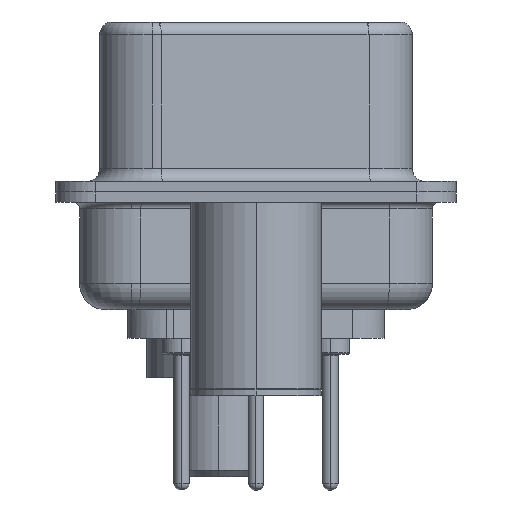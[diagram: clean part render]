
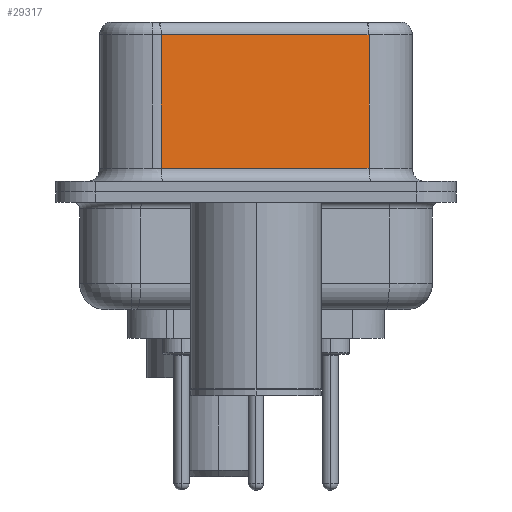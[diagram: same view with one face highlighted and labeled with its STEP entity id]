
A CAD part, left-side view. The second image highlights one B-rep face of the part: STEP entity #29317.
In plain terms, the highlighted planar face has unit normal (-0.985, -0.174, 0).
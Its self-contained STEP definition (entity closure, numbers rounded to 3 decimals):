
#489 = EDGE_CURVE ( 'NONE', #21842, #25849, #25945, .T. ) ;
#1246 = LINE ( 'NONE', #29912, #21366 ) ;
#1677 = ORIENTED_EDGE ( 'NONE', *, *, #489, .T. ) ;
#4131 = CARTESIAN_POINT ( 'NONE',  ( 5.132, -4.322, 6.52 ) ) ;
#5094 = VECTOR ( 'NONE', #27784, 1000. ) ;
#6689 = PLANE ( 'NONE',  #12031 ) ;
#7883 = DIRECTION ( 'NONE',  ( -0.174, 0.985, 0. ) ) ;
#8795 = ORIENTED_EDGE ( 'NONE', *, *, #30338, .T. ) ;
#10696 = EDGE_LOOP ( 'NONE', ( #17632, #11243, #1677, #8795 ) ) ;
#11243 = ORIENTED_EDGE ( 'NONE', *, *, #29859, .T. ) ;
#11762 = DIRECTION ( 'NONE',  ( -0.174, 0.985, 0. ) ) ;
#12031 = AXIS2_PLACEMENT_3D ( 'NONE', #4131, #26815, #11762 ) ;
#12328 = DIRECTION ( 'NONE',  ( 0.174, -0.985, 0. ) ) ;
#12344 = VECTOR ( 'NONE', #7883, 1000. ) ;
#14099 = DIRECTION ( 'NONE',  ( 0., 0., -1. ) ) ;
#14786 = VECTOR ( 'NONE', #14099, 1000. ) ;
#14796 = CARTESIAN_POINT ( 'NONE',  ( 3.73, 3.628, 0.9 ) ) ;
#17632 = ORIENTED_EDGE ( 'NONE', *, *, #28607, .F. ) ;
#17885 = CARTESIAN_POINT ( 'NONE',  ( 3.73, 3.628, 6.02 ) ) ;
#18937 = VERTEX_POINT ( 'NONE', #21429 ) ;
#19821 = LINE ( 'NONE', #27975, #12344 ) ;
#21366 = VECTOR ( 'NONE', #12328, 1000. ) ;
#21429 = CARTESIAN_POINT ( 'NONE',  ( 5.132, -4.322, 0.9 ) ) ;
#21842 = VERTEX_POINT ( 'NONE', #17885 ) ;
#22849 = CARTESIAN_POINT ( 'NONE',  ( 3.73, 3.628, 6.52 ) ) ;
#25738 = FACE_OUTER_BOUND ( 'NONE', #10696, .T. ) ;
#25849 = VERTEX_POINT ( 'NONE', #14796 ) ;
#25945 = LINE ( 'NONE', #22849, #5094 ) ;
#26815 = DIRECTION ( 'NONE',  ( 0.985, 0.174, 0. ) ) ;
#27784 = DIRECTION ( 'NONE',  ( 0., 0., -1. ) ) ;
#27975 = CARTESIAN_POINT ( 'NONE',  ( 5.132, -4.322, 6.02 ) ) ;
#28164 = LINE ( 'NONE', #31644, #14786 ) ;
#28274 = CARTESIAN_POINT ( 'NONE',  ( 5.132, -4.322, 6.02 ) ) ;
#28607 = EDGE_CURVE ( 'NONE', #29070, #18937, #28164, .T. ) ;
#29070 = VERTEX_POINT ( 'NONE', #28274 ) ;
#29317 = ADVANCED_FACE ( 'NONE', ( #25738 ), #6689, .F. ) ;
#29859 = EDGE_CURVE ( 'NONE', #29070, #21842, #19821, .T. ) ;
#29912 = CARTESIAN_POINT ( 'NONE',  ( 5.132, -4.322, 0.9 ) ) ;
#30338 = EDGE_CURVE ( 'NONE', #25849, #18937, #1246, .T. ) ;
#31644 = CARTESIAN_POINT ( 'NONE',  ( 5.132, -4.322, 6.52 ) ) ;
